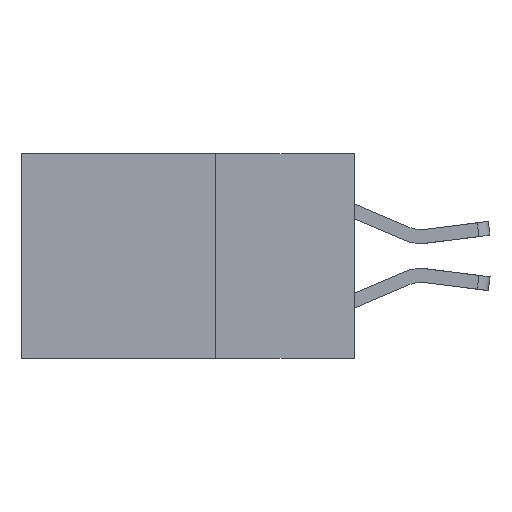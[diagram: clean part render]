
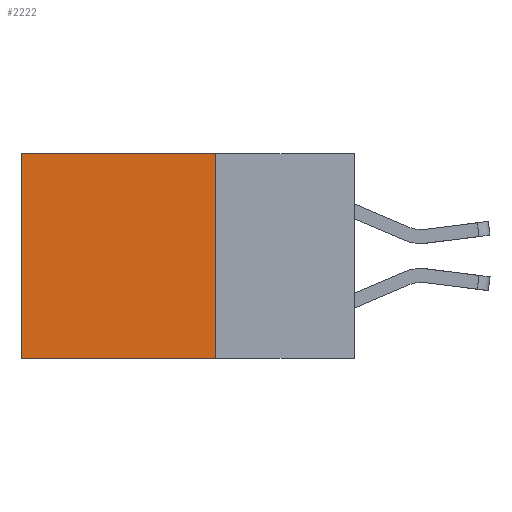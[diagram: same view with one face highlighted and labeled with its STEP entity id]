
A CAD part, left-side view. The second image highlights one B-rep face of the part: STEP entity #2222.
In plain terms, the highlighted planar face has unit normal (-1, 0, 0).
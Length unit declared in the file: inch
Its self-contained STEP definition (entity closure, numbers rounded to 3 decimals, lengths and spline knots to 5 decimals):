
#54 = CARTESIAN_POINT ( 'NONE',  ( 0.2615, 0.6, 0. ) ) ;
#265 = LINE ( 'NONE', #4834, #8927 ) ;
#555 = VECTOR ( 'NONE', #9029, 39.37008 ) ;
#1150 = ORIENTED_EDGE ( 'NONE', *, *, #6786, .F. ) ;
#1259 = CARTESIAN_POINT ( 'NONE',  ( 0.2615, 0.25, -0.37 ) ) ;
#1392 = VERTEX_POINT ( 'NONE', #9926 ) ;
#1428 = LINE ( 'NONE', #1259, #9835 ) ;
#1915 = AXIS2_PLACEMENT_3D ( 'NONE', #4382, #6991, #6028 ) ;
#2222 = ADVANCED_FACE ( 'NONE', ( #2978 ), #4254, .F. ) ;
#2299 = DIRECTION ( 'NONE',  ( 0., 1., 0. ) ) ;
#2401 = CARTESIAN_POINT ( 'NONE',  ( 0.2615, 0.25, -0.37 ) ) ;
#2978 = FACE_OUTER_BOUND ( 'NONE', #6712, .T. ) ;
#4254 = PLANE ( 'NONE',  #1915 ) ;
#4268 = VECTOR ( 'NONE', #9860, 39.37008 ) ;
#4382 = CARTESIAN_POINT ( 'NONE',  ( 0.2615, 0.25, -0.37 ) ) ;
#4483 = EDGE_CURVE ( 'NONE', #8674, #9349, #7249, .T. ) ;
#4690 = ORIENTED_EDGE ( 'NONE', *, *, #4938, .T. ) ;
#4834 = CARTESIAN_POINT ( 'NONE',  ( 0.2615, 0.25, -0.37 ) ) ;
#4938 = EDGE_CURVE ( 'NONE', #9349, #1392, #9387, .T. ) ;
#5188 = CARTESIAN_POINT ( 'NONE',  ( 0.2615, 0.25, 0. ) ) ;
#5443 = VERTEX_POINT ( 'NONE', #2401 ) ;
#6028 = DIRECTION ( 'NONE',  ( 0., 0., -1. ) ) ;
#6435 = ORIENTED_EDGE ( 'NONE', *, *, #6709, .F. ) ;
#6709 = EDGE_CURVE ( 'NONE', #8674, #5443, #1428, .T. ) ;
#6712 = EDGE_LOOP ( 'NONE', ( #4690, #1150, #6435, #7509 ) ) ;
#6786 = EDGE_CURVE ( 'NONE', #5443, #1392, #265, .T. ) ;
#6991 = DIRECTION ( 'NONE',  ( 1., 0., 0. ) ) ;
#7210 = DIRECTION ( 'NONE',  ( 0., 0., -1. ) ) ;
#7249 = LINE ( 'NONE', #5188, #4268 ) ;
#7509 = ORIENTED_EDGE ( 'NONE', *, *, #4483, .T. ) ;
#8674 = VERTEX_POINT ( 'NONE', #8712 ) ;
#8712 = CARTESIAN_POINT ( 'NONE',  ( 0.2615, 0.25, 0. ) ) ;
#8927 = VECTOR ( 'NONE', #2299, 39.37008 ) ;
#9029 = DIRECTION ( 'NONE',  ( 0., 0., -1. ) ) ;
#9349 = VERTEX_POINT ( 'NONE', #54 ) ;
#9387 = LINE ( 'NONE', #9727, #555 ) ;
#9727 = CARTESIAN_POINT ( 'NONE',  ( 0.2615, 0.6, -0.37 ) ) ;
#9835 = VECTOR ( 'NONE', #7210, 39.37008 ) ;
#9860 = DIRECTION ( 'NONE',  ( 0., 1., 0. ) ) ;
#9926 = CARTESIAN_POINT ( 'NONE',  ( 0.2615, 0.6, -0.37 ) ) ;
